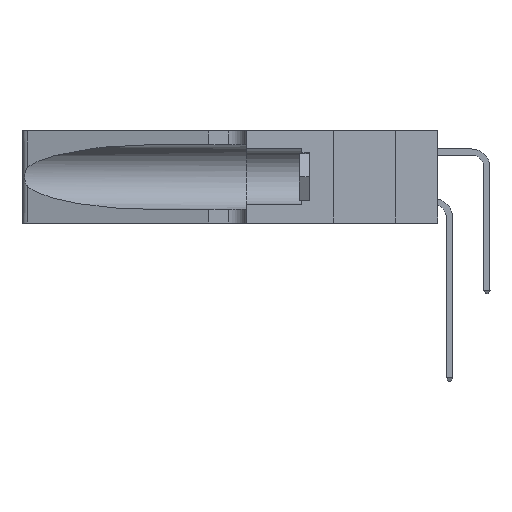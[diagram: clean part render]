
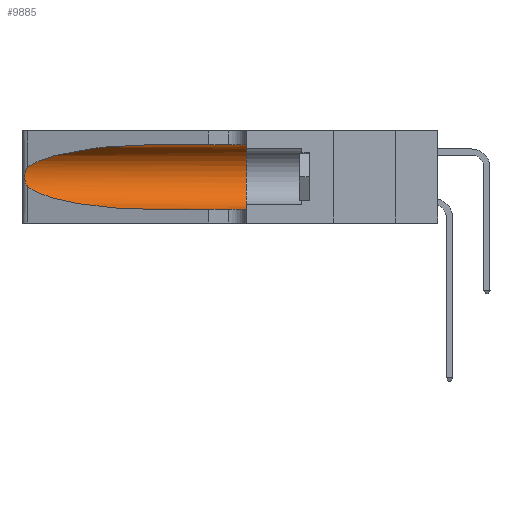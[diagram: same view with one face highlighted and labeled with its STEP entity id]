
A CAD part, left-side view. The second image highlights one B-rep face of the part: STEP entity #9885.
In plain terms, the highlighted cylindrical face has radius 3.308 mm (diameter 6.617 mm), a partial arc.
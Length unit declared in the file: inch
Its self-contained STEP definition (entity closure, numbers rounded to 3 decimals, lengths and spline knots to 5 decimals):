
#175 = CARTESIAN_POINT ( 'NONE',  ( 0.18966, 0.96281, 0.05475 ) ) ;
#624 = AXIS2_PLACEMENT_3D ( 'NONE', #10706, #8921, #23254 ) ;
#889 = CARTESIAN_POINT ( 'NONE',  ( 0.25487, 1.22718, 0.22369 ) ) ;
#970 = CARTESIAN_POINT ( 'NONE',  ( 0.25789, 1.23486, 0.15765 ) ) ;
#2725 = CARTESIAN_POINT ( 'NONE',  ( 0.25555, 1.22994, 0.2215 ) ) ;
#2804 = CARTESIAN_POINT ( 'NONE',  ( 0.25555, 1.22993, 0.14849 ) ) ;
#3090 = VERTEX_POINT ( 'NONE', #7342 ) ;
#3624 = ORIENTED_EDGE ( 'NONE', *, *, #8699, .T. ) ;
#3674 = B_SPLINE_CURVE_WITH_KNOTS ( 'NONE', 3,
 ( #889, #2725, #17121, #6334, #18880, #8160, #20693, #9949, #22504, #11764, #970, #13579, #2804, #15386 ),
 .UNSPECIFIED., .F., .F.,
 ( 4, 2, 2, 2, 2, 2, 4 ),
 ( 0., 0.00027, 0.00053, 0.00107, 0.0016, 0.00187, 0.00214 ),
 .UNSPECIFIED. ) ;
#5020 = CIRCLE ( 'NONE', #19331, 0.13025 ) ;
#5391 =( BOUNDED_CURVE ( )  B_SPLINE_CURVE ( 3, ( #7343, #18110, #175, #12777 ),
 .UNSPECIFIED., .F., .F. ) 
 B_SPLINE_CURVE_WITH_KNOTS ( ( 4, 4 ),
 ( 3.44316, 4.71239 ),
 .UNSPECIFIED. ) 
 CURVE ( )  GEOMETRIC_REPRESENTATION_ITEM ( )  RATIONAL_B_SPLINE_CURVE ( ( 1., 0.87, 0.87, 1. ) ) 
 REPRESENTATION_ITEM ( '' )  );
#5646 = CARTESIAN_POINT ( 'NONE',  ( 0.1305, 0.35, 0.31525 ) ) ;
#6334 = CARTESIAN_POINT ( 'NONE',  ( 0.25787, 1.23484, 0.2124 ) ) ;
#6427 = EDGE_CURVE ( 'NONE', #12361, #15755, #18630, .T. ) ;
#6788 = CARTESIAN_POINT ( 'NONE',  ( 0.1305, 0.35, 0.05475 ) ) ;
#7025 = ORIENTED_EDGE ( 'NONE', *, *, #20823, .F. ) ;
#7177 = EDGE_CURVE ( 'NONE', #12586, #3090, #5391, .T. ) ;
#7342 = CARTESIAN_POINT ( 'NONE',  ( 0.1305, 0.72297, 0.05475 ) ) ;
#7343 = CARTESIAN_POINT ( 'NONE',  ( 0.25487, 1.22718, 0.14631 ) ) ;
#7500 = VERTEX_POINT ( 'NONE', #6788 ) ;
#7627 = ORIENTED_EDGE ( 'NONE', *, *, #6427, .F. ) ;
#8160 = CARTESIAN_POINT ( 'NONE',  ( 0.26018, 1.23835, 0.19895 ) ) ;
#8641 = ORIENTED_EDGE ( 'NONE', *, *, #7177, .T. ) ;
#8699 = EDGE_CURVE ( 'NONE', #3090, #7500, #18375, .T. ) ;
#8921 = DIRECTION ( 'NONE',  ( 0., -1., 0. ) ) ;
#9284 = CARTESIAN_POINT ( 'NONE',  ( 0.1305, 0.35, 0.185 ) ) ;
#9659 = VECTOR ( 'NONE', #14921, 39.37008 ) ;
#9885 = ADVANCED_FACE ( 'NONE', ( #18059 ), #16955, .F. ) ;
#9949 = CARTESIAN_POINT ( 'NONE',  ( 0.26075, 1.23896, 0.178 ) ) ;
#10706 = CARTESIAN_POINT ( 'NONE',  ( 0.1305, 1.61858, 0.185 ) ) ;
#10750 = CARTESIAN_POINT ( 'NONE',  ( 0.1305, 1.61858, 0.31525 ) ) ;
#10840 = CARTESIAN_POINT ( 'NONE',  ( 0.1305, 1.61858, 0.05475 ) ) ;
#10917 = EDGE_CURVE ( 'NONE', #13090, #12586, #3674, .T. ) ;
#11090 = DIRECTION ( 'NONE',  ( 0., 0., 1. ) ) ;
#11655 = EDGE_CURVE ( 'NONE', #12361, #13090, #18607, .T. ) ;
#11764 = CARTESIAN_POINT ( 'NONE',  ( 0.25856, 1.23593, 0.16098 ) ) ;
#12212 = CARTESIAN_POINT ( 'NONE',  ( 0.25487, 1.22718, 0.22369 ) ) ;
#12361 = VERTEX_POINT ( 'NONE', #17752 ) ;
#12586 = VERTEX_POINT ( 'NONE', #20128 ) ;
#12777 = CARTESIAN_POINT ( 'NONE',  ( 0.1305, 0.72297, 0.05475 ) ) ;
#13090 = VERTEX_POINT ( 'NONE', #21536 ) ;
#13092 = EDGE_LOOP ( 'NONE', ( #15769, #17900, #8641, #3624, #7025, #7627 ) ) ;
#13579 = CARTESIAN_POINT ( 'NONE',  ( 0.25639, 1.23186, 0.15144 ) ) ;
#14470 = DIRECTION ( 'NONE',  ( 0., -1., 0. ) ) ;
#14921 = DIRECTION ( 'NONE',  ( 0., -1., 0. ) ) ;
#15386 = CARTESIAN_POINT ( 'NONE',  ( 0.25487, 1.22718, 0.14631 ) ) ;
#15755 = VERTEX_POINT ( 'NONE', #5646 ) ;
#15769 = ORIENTED_EDGE ( 'NONE', *, *, #11655, .T. ) ;
#16955 = CYLINDRICAL_SURFACE ( 'NONE', #624, 0.13025 ) ;
#17121 = CARTESIAN_POINT ( 'NONE',  ( 0.25639, 1.23184, 0.21858 ) ) ;
#17752 = CARTESIAN_POINT ( 'NONE',  ( 0.1305, 0.72297, 0.31525 ) ) ;
#17900 = ORIENTED_EDGE ( 'NONE', *, *, #10917, .T. ) ;
#18059 = FACE_OUTER_BOUND ( 'NONE', #13092, .T. ) ;
#18110 = CARTESIAN_POINT ( 'NONE',  ( 0.2373, 1.15595, 0.08982 ) ) ;
#18375 = LINE ( 'NONE', #10840, #22588 ) ;
#18607 =( BOUNDED_CURVE ( )  B_SPLINE_CURVE ( 3, ( #19319, #21060, #22937, #12212 ),
 .UNSPECIFIED., .F., .F. ) 
 B_SPLINE_CURVE_WITH_KNOTS ( ( 4, 4 ),
 ( 1.5708, 2.84003 ),
 .UNSPECIFIED. ) 
 CURVE ( )  GEOMETRIC_REPRESENTATION_ITEM ( )  RATIONAL_B_SPLINE_CURVE ( ( 1., 0.87, 0.87, 1. ) ) 
 REPRESENTATION_ITEM ( '' )  );
#18630 = LINE ( 'NONE', #10750, #9659 ) ;
#18880 = CARTESIAN_POINT ( 'NONE',  ( 0.25854, 1.2359, 0.20912 ) ) ;
#19319 = CARTESIAN_POINT ( 'NONE',  ( 0.1305, 0.72297, 0.31525 ) ) ;
#19331 = AXIS2_PLACEMENT_3D ( 'NONE', #9284, #21819, #11090 ) ;
#20128 = CARTESIAN_POINT ( 'NONE',  ( 0.25487, 1.22718, 0.14631 ) ) ;
#20693 = CARTESIAN_POINT ( 'NONE',  ( 0.26075, 1.23896, 0.19203 ) ) ;
#20823 = EDGE_CURVE ( 'NONE', #15755, #7500, #5020, .T. ) ;
#21060 = CARTESIAN_POINT ( 'NONE',  ( 0.18966, 0.96281, 0.31525 ) ) ;
#21536 = CARTESIAN_POINT ( 'NONE',  ( 0.25487, 1.22718, 0.22369 ) ) ;
#21819 = DIRECTION ( 'NONE',  ( 0., 1., 0. ) ) ;
#22504 = CARTESIAN_POINT ( 'NONE',  ( 0.26017, 1.23833, 0.17102 ) ) ;
#22588 = VECTOR ( 'NONE', #14470, 39.37008 ) ;
#22937 = CARTESIAN_POINT ( 'NONE',  ( 0.2373, 1.15595, 0.28018 ) ) ;
#23254 = DIRECTION ( 'NONE',  ( 0., 0., -1. ) ) ;
